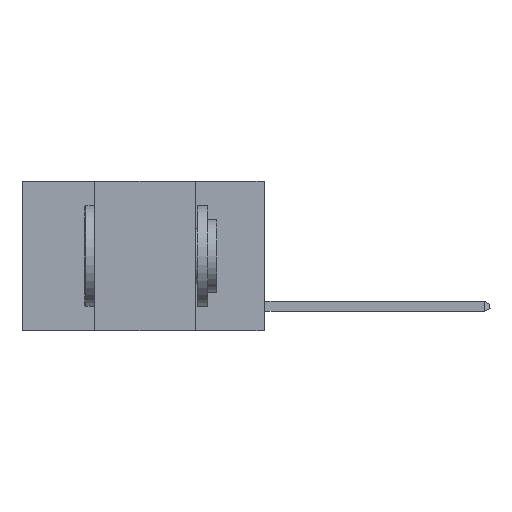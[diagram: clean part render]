
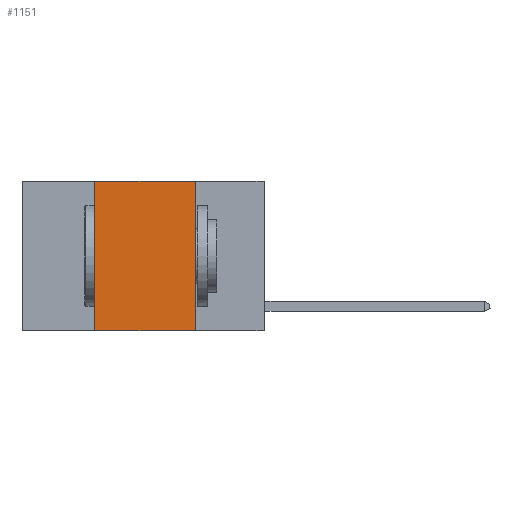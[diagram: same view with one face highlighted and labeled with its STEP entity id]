
A CAD part, left-side view. The second image highlights one B-rep face of the part: STEP entity #1151.
In plain terms, the highlighted planar face has unit normal (-1, 0, 0).
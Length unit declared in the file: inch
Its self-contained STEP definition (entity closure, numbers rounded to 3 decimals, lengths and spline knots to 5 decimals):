
#183 = DIRECTION ( 'NONE',  ( 0., -1., 0. ) ) ;
#593 = ORIENTED_EDGE ( 'NONE', *, *, #6565, .T. ) ;
#914 = VECTOR ( 'NONE', #9496, 39.37008 ) ;
#1151 = ADVANCED_FACE ( 'NONE', ( #12135 ), #2004, .F. ) ;
#1221 = CARTESIAN_POINT ( 'NONE',  ( 0., 0.17, 0. ) ) ;
#2004 = PLANE ( 'NONE',  #13873 ) ;
#2553 = VECTOR ( 'NONE', #9987, 39.37008 ) ;
#2753 = CARTESIAN_POINT ( 'NONE',  ( 0., 0.42, 0. ) ) ;
#3062 = CARTESIAN_POINT ( 'NONE',  ( 0., 0.42, -0.37 ) ) ;
#3626 = EDGE_LOOP ( 'NONE', ( #4640, #11549, #9807, #593 ) ) ;
#4186 = CARTESIAN_POINT ( 'NONE',  ( 0., 0.17, 0. ) ) ;
#4640 = ORIENTED_EDGE ( 'NONE', *, *, #6541, .F. ) ;
#5904 = CARTESIAN_POINT ( 'NONE',  ( 0., 0.6, 0. ) ) ;
#6539 = CARTESIAN_POINT ( 'NONE',  ( 0., 0.6, 0. ) ) ;
#6541 = EDGE_CURVE ( 'NONE', #8687, #13316, #9017, .T. ) ;
#6565 = EDGE_CURVE ( 'NONE', #13092, #13316, #6933, .T. ) ;
#6686 = EDGE_CURVE ( 'NONE', #13092, #14065, #8385, .T. ) ;
#6933 = LINE ( 'NONE', #13751, #914 ) ;
#7414 = DIRECTION ( 'NONE',  ( 0., 0., -1. ) ) ;
#7474 = CARTESIAN_POINT ( 'NONE',  ( 0., 0.42, 0. ) ) ;
#7880 = EDGE_CURVE ( 'NONE', #14065, #8687, #12769, .T. ) ;
#8385 = LINE ( 'NONE', #2753, #8482 ) ;
#8482 = VECTOR ( 'NONE', #12489, 39.37008 ) ;
#8687 = VERTEX_POINT ( 'NONE', #1221 ) ;
#9017 = LINE ( 'NONE', #4186, #2553 ) ;
#9496 = DIRECTION ( 'NONE',  ( 0., -1., 0. ) ) ;
#9801 = DIRECTION ( 'NONE',  ( 1., 0., 0. ) ) ;
#9807 = ORIENTED_EDGE ( 'NONE', *, *, #6686, .F. ) ;
#9987 = DIRECTION ( 'NONE',  ( 0., 0., -1. ) ) ;
#11549 = ORIENTED_EDGE ( 'NONE', *, *, #7880, .F. ) ;
#12135 = FACE_OUTER_BOUND ( 'NONE', #3626, .T. ) ;
#12489 = DIRECTION ( 'NONE',  ( 0., 0., 1. ) ) ;
#12769 = LINE ( 'NONE', #5904, #14152 ) ;
#13092 = VERTEX_POINT ( 'NONE', #3062 ) ;
#13316 = VERTEX_POINT ( 'NONE', #13587 ) ;
#13587 = CARTESIAN_POINT ( 'NONE',  ( 0., 0.17, -0.37 ) ) ;
#13751 = CARTESIAN_POINT ( 'NONE',  ( 0., 0.6, -0.37 ) ) ;
#13873 = AXIS2_PLACEMENT_3D ( 'NONE', #6539, #9801, #7414 ) ;
#14065 = VERTEX_POINT ( 'NONE', #7474 ) ;
#14152 = VECTOR ( 'NONE', #183, 39.37008 ) ;
